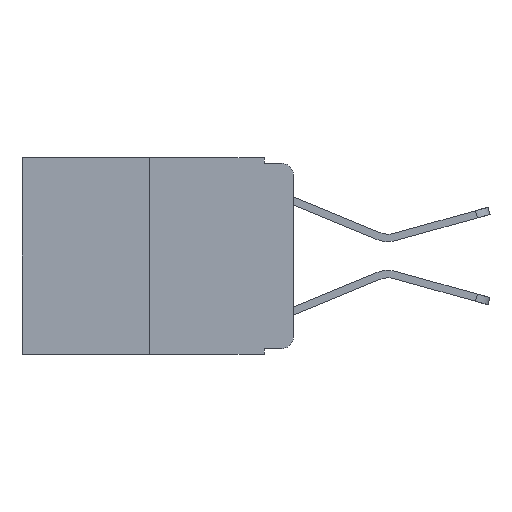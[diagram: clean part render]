
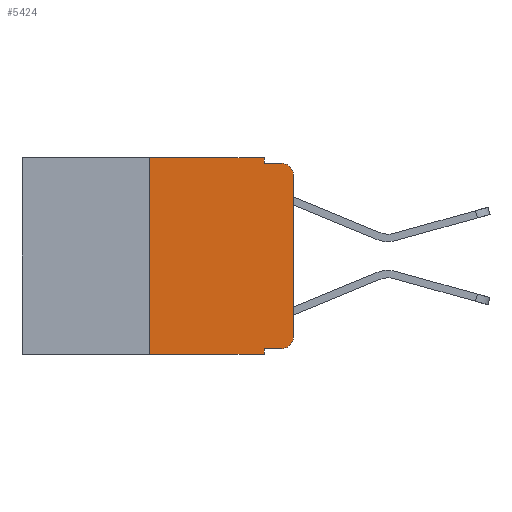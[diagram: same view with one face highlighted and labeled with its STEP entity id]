
A CAD part, left-side view. The second image highlights one B-rep face of the part: STEP entity #5424.
In plain terms, the highlighted planar face has unit normal (-1, 0, 0).
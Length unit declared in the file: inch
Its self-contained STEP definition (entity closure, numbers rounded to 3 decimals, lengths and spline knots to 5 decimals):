
#32 = CARTESIAN_POINT ( 'NONE',  ( 0., 0.051, 0. ) ) ;
#122 = CARTESIAN_POINT ( 'NONE',  ( 0., 0., -0.313 ) ) ;
#222 = ORIENTED_EDGE ( 'NONE', *, *, #4625, .F. ) ;
#239 = EDGE_CURVE ( 'NONE', #854, #2777, #9016, .T. ) ;
#409 = DIRECTION ( 'NONE',  ( -1., 0., 0. ) ) ;
#695 = ORIENTED_EDGE ( 'NONE', *, *, #239, .T. ) ;
#854 = VERTEX_POINT ( 'NONE', #10815 ) ;
#1051 = EDGE_CURVE ( 'NONE', #3650, #854, #1115, .T. ) ;
#1089 = ORIENTED_EDGE ( 'NONE', *, *, #1051, .T. ) ;
#1115 = LINE ( 'NONE', #8084, #11408 ) ;
#1123 = AXIS2_PLACEMENT_3D ( 'NONE', #5480, #6489, #10289 ) ;
#1563 = CARTESIAN_POINT ( 'NONE',  ( 0., 0.051, -0.333 ) ) ;
#2058 = EDGE_LOOP ( 'NONE', ( #5028, #5161, #3999, #5893, #6687, #5304, #4923, #222, #1089, #695 ) ) ;
#2777 = VERTEX_POINT ( 'NONE', #122 ) ;
#2901 = PLANE ( 'NONE',  #3575 ) ;
#3464 = VERTEX_POINT ( 'NONE', #4437 ) ;
#3531 = VERTEX_POINT ( 'NONE', #9386 ) ;
#3575 = AXIS2_PLACEMENT_3D ( 'NONE', #5889, #12583, #6862 ) ;
#3650 = VERTEX_POINT ( 'NONE', #1563 ) ;
#3736 = DIRECTION ( 'NONE',  ( 0., 0., 1. ) ) ;
#3841 = CARTESIAN_POINT ( 'NONE',  ( 0., 0., 0. ) ) ;
#3999 = ORIENTED_EDGE ( 'NONE', *, *, #8574, .F. ) ;
#4108 = VECTOR ( 'NONE', #4962, 39.37008 ) ;
#4358 = CARTESIAN_POINT ( 'NONE',  ( 0., 0.02, -0.01 ) ) ;
#4433 = FACE_OUTER_BOUND ( 'NONE', #2058, .T. ) ;
#4437 = CARTESIAN_POINT ( 'NONE',  ( 0., 0.051, -0.01 ) ) ;
#4625 = EDGE_CURVE ( 'NONE', #3650, #6522, #9192, .T. ) ;
#4923 = ORIENTED_EDGE ( 'NONE', *, *, #6778, .T. ) ;
#4962 = DIRECTION ( 'NONE',  ( 0., -1., 0. ) ) ;
#5028 = ORIENTED_EDGE ( 'NONE', *, *, #9837, .T. ) ;
#5161 = ORIENTED_EDGE ( 'NONE', *, *, #9213, .T. ) ;
#5296 = EDGE_CURVE ( 'NONE', #9817, #3531, #7660, .T. ) ;
#5304 = ORIENTED_EDGE ( 'NONE', *, *, #5296, .F. ) ;
#5353 = VECTOR ( 'NONE', #6418, 39.37008 ) ;
#5365 = VECTOR ( 'NONE', #3736, 39.37008 ) ;
#5424 = ADVANCED_FACE ( 'NONE', ( #4433 ), #2901, .F. ) ;
#5480 = CARTESIAN_POINT ( 'NONE',  ( 0., 0.02, -0.313 ) ) ;
#5889 = CARTESIAN_POINT ( 'NONE',  ( 0., 0.473, 0. ) ) ;
#5893 = ORIENTED_EDGE ( 'NONE', *, *, #5957, .F. ) ;
#5957 = EDGE_CURVE ( 'NONE', #7749, #3464, #9893, .T. ) ;
#6230 = DIRECTION ( 'NONE',  ( 0., -1., 0. ) ) ;
#6418 = DIRECTION ( 'NONE',  ( 0., 0., -1. ) ) ;
#6489 = DIRECTION ( 'NONE',  ( -1., 0., 0. ) ) ;
#6522 = VERTEX_POINT ( 'NONE', #9082 ) ;
#6623 = VECTOR ( 'NONE', #11179, 39.37008 ) ;
#6683 = DIRECTION ( 'NONE',  ( 0., -1., 0. ) ) ;
#6685 = CARTESIAN_POINT ( 'NONE',  ( 0., 0.02, -0.03 ) ) ;
#6687 = ORIENTED_EDGE ( 'NONE', *, *, #11841, .F. ) ;
#6758 = CARTESIAN_POINT ( 'NONE',  ( 0., 0.051, 0. ) ) ;
#6778 = EDGE_CURVE ( 'NONE', #9817, #6522, #7255, .T. ) ;
#6862 = DIRECTION ( 'NONE',  ( 0., 0., -1. ) ) ;
#7255 = LINE ( 'NONE', #9548, #12018 ) ;
#7660 = LINE ( 'NONE', #10510, #5365 ) ;
#7676 = DIRECTION ( 'NONE',  ( 0., 0., -1. ) ) ;
#7749 = VERTEX_POINT ( 'NONE', #12452 ) ;
#8084 = CARTESIAN_POINT ( 'NONE',  ( 0., 0.051, -0.333 ) ) ;
#8101 = CIRCLE ( 'NONE', #9718, 0.02 ) ;
#8574 = EDGE_CURVE ( 'NONE', #3464, #10219, #11519, .T. ) ;
#8892 = VECTOR ( 'NONE', #9661, 39.37008 ) ;
#9016 = CIRCLE ( 'NONE', #1123, 0.02 ) ;
#9082 = CARTESIAN_POINT ( 'NONE',  ( 0., 0.051, -0.343 ) ) ;
#9192 = LINE ( 'NONE', #6758, #8892 ) ;
#9213 = EDGE_CURVE ( 'NONE', #12040, #10219, #8101, .T. ) ;
#9268 = CARTESIAN_POINT ( 'NONE',  ( 0., 0.473, 0. ) ) ;
#9386 = CARTESIAN_POINT ( 'NONE',  ( 0., 0.25, 0. ) ) ;
#9417 = VECTOR ( 'NONE', #10606, 39.37008 ) ;
#9479 = LINE ( 'NONE', #9268, #6623 ) ;
#9548 = CARTESIAN_POINT ( 'NONE',  ( 0., 0.473, -0.343 ) ) ;
#9661 = DIRECTION ( 'NONE',  ( 0., 0., -1. ) ) ;
#9718 = AXIS2_PLACEMENT_3D ( 'NONE', #6685, #409, #7676 ) ;
#9796 = CARTESIAN_POINT ( 'NONE',  ( 0., 0.051, -0.01 ) ) ;
#9817 = VERTEX_POINT ( 'NONE', #12487 ) ;
#9837 = EDGE_CURVE ( 'NONE', #2777, #12040, #12225, .T. ) ;
#9893 = LINE ( 'NONE', #32, #5353 ) ;
#10219 = VERTEX_POINT ( 'NONE', #4358 ) ;
#10289 = DIRECTION ( 'NONE',  ( 0., 0., -1. ) ) ;
#10510 = CARTESIAN_POINT ( 'NONE',  ( 0., 0.25, 0. ) ) ;
#10606 = DIRECTION ( 'NONE',  ( 0., 0., 1. ) ) ;
#10815 = CARTESIAN_POINT ( 'NONE',  ( 0., 0.02, -0.333 ) ) ;
#10848 = CARTESIAN_POINT ( 'NONE',  ( 0., 0., -0.03 ) ) ;
#11179 = DIRECTION ( 'NONE',  ( 0., -1., 0. ) ) ;
#11408 = VECTOR ( 'NONE', #6230, 39.37008 ) ;
#11519 = LINE ( 'NONE', #9796, #4108 ) ;
#11841 = EDGE_CURVE ( 'NONE', #3531, #7749, #9479, .T. ) ;
#12018 = VECTOR ( 'NONE', #6683, 39.37008 ) ;
#12040 = VERTEX_POINT ( 'NONE', #10848 ) ;
#12225 = LINE ( 'NONE', #3841, #9417 ) ;
#12452 = CARTESIAN_POINT ( 'NONE',  ( 0., 0.051, 0. ) ) ;
#12487 = CARTESIAN_POINT ( 'NONE',  ( 0., 0.25, -0.343 ) ) ;
#12583 = DIRECTION ( 'NONE',  ( 1., 0., 0. ) ) ;
